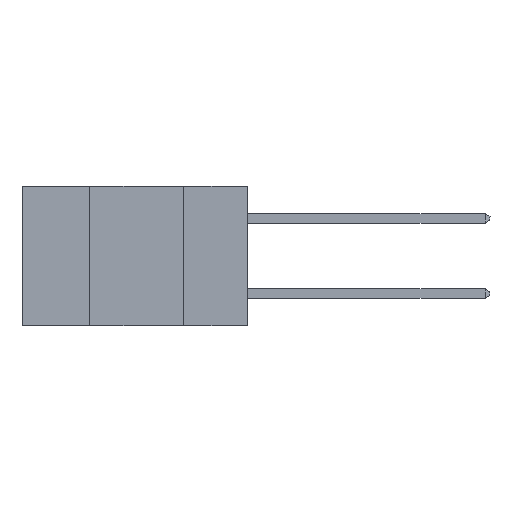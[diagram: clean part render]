
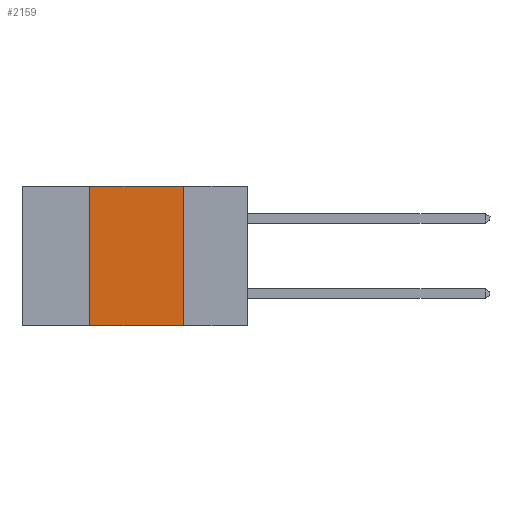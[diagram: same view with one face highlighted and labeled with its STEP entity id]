
A CAD part, left-side view. The second image highlights one B-rep face of the part: STEP entity #2159.
In plain terms, the highlighted planar face has unit normal (-1, 0, 0).
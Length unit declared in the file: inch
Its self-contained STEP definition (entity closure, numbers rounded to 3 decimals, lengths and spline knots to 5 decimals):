
#113 = CARTESIAN_POINT ( 'NONE',  ( 0., 0.42, -0.37 ) ) ;
#576 = AXIS2_PLACEMENT_3D ( 'NONE', #4969, #7469, #2049 ) ;
#1686 = LINE ( 'NONE', #6227, #5718 ) ;
#1770 = ORIENTED_EDGE ( 'NONE', *, *, #2703, .T. ) ;
#1823 = VERTEX_POINT ( 'NONE', #8394 ) ;
#2013 = EDGE_CURVE ( 'NONE', #6085, #7140, #4096, .T. ) ;
#2049 = DIRECTION ( 'NONE',  ( 0., 0., -1. ) ) ;
#2159 = ADVANCED_FACE ( 'NONE', ( #9123 ), #9707, .F. ) ;
#2232 = ORIENTED_EDGE ( 'NONE', *, *, #5185, .F. ) ;
#2278 = EDGE_CURVE ( 'NONE', #1823, #6085, #6871, .T. ) ;
#2586 = DIRECTION ( 'NONE',  ( 0., -1., 0. ) ) ;
#2703 = EDGE_CURVE ( 'NONE', #5936, #7140, #1686, .T. ) ;
#3559 = VECTOR ( 'NONE', #2586, 39.37008 ) ;
#3929 = CARTESIAN_POINT ( 'NONE',  ( 0., 0.6, 0. ) ) ;
#4096 = LINE ( 'NONE', #7091, #7279 ) ;
#4969 = CARTESIAN_POINT ( 'NONE',  ( 0., 0.6, 0. ) ) ;
#5185 = EDGE_CURVE ( 'NONE', #5936, #1823, #5341, .T. ) ;
#5339 = DIRECTION ( 'NONE',  ( 0., -1., 0. ) ) ;
#5341 = LINE ( 'NONE', #113, #9163 ) ;
#5628 = CARTESIAN_POINT ( 'NONE',  ( 0., 0.17, -0.37 ) ) ;
#5718 = VECTOR ( 'NONE', #5339, 39.37008 ) ;
#5936 = VERTEX_POINT ( 'NONE', #6097 ) ;
#6085 = VERTEX_POINT ( 'NONE', #7722 ) ;
#6097 = CARTESIAN_POINT ( 'NONE',  ( 0., 0.42, -0.37 ) ) ;
#6227 = CARTESIAN_POINT ( 'NONE',  ( 0., 0.6, -0.37 ) ) ;
#6269 = DIRECTION ( 'NONE',  ( 0., 0., 1. ) ) ;
#6871 = LINE ( 'NONE', #3929, #3559 ) ;
#7048 = ORIENTED_EDGE ( 'NONE', *, *, #2013, .F. ) ;
#7091 = CARTESIAN_POINT ( 'NONE',  ( 0., 0.17, -0.37 ) ) ;
#7140 = VERTEX_POINT ( 'NONE', #5628 ) ;
#7279 = VECTOR ( 'NONE', #7839, 39.37008 ) ;
#7469 = DIRECTION ( 'NONE',  ( 1., 0., 0. ) ) ;
#7606 = EDGE_LOOP ( 'NONE', ( #7048, #8710, #2232, #1770 ) ) ;
#7722 = CARTESIAN_POINT ( 'NONE',  ( 0., 0.17, 0. ) ) ;
#7839 = DIRECTION ( 'NONE',  ( 0., 0., -1. ) ) ;
#8394 = CARTESIAN_POINT ( 'NONE',  ( 0., 0.42, 0. ) ) ;
#8710 = ORIENTED_EDGE ( 'NONE', *, *, #2278, .F. ) ;
#9123 = FACE_OUTER_BOUND ( 'NONE', #7606, .T. ) ;
#9163 = VECTOR ( 'NONE', #6269, 39.37008 ) ;
#9707 = PLANE ( 'NONE',  #576 ) ;
